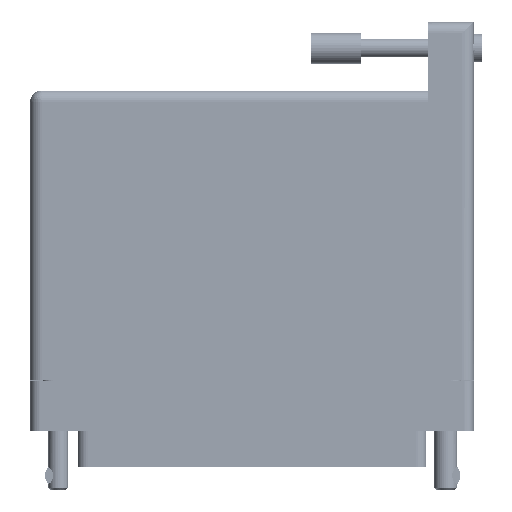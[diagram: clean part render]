
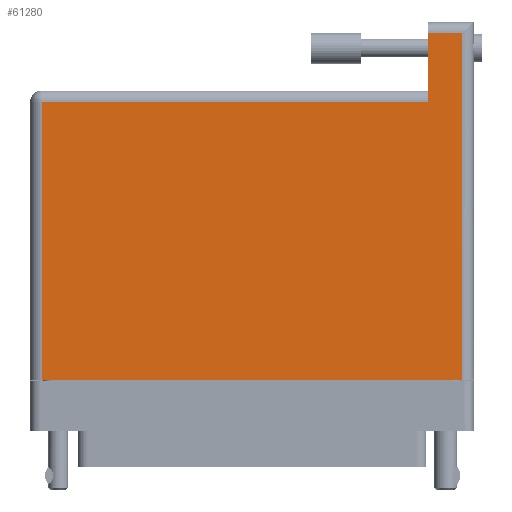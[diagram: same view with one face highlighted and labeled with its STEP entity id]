
A CAD part, front view. The second image highlights one B-rep face of the part: STEP entity #61280.
In plain terms, the highlighted face is planar.
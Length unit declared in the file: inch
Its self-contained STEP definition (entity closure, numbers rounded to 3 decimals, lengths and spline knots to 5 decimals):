
#1107 = VECTOR ( 'NONE', #55226, 39.37008 ) ;
#3086 = FACE_OUTER_BOUND ( 'NONE', #18941, .T. ) ;
#3192 = CARTESIAN_POINT ( 'NONE',  ( -1.359, 2.025, 0.617 ) ) ;
#4918 = DIRECTION ( 'NONE',  ( 1., 0., 0. ) ) ;
#5148 = LINE ( 'NONE', #23164, #1107 ) ;
#5359 = EDGE_CURVE ( 'NONE', #36447, #42896, #19551, .T. ) ;
#5602 = CARTESIAN_POINT ( 'NONE',  ( 1.289, 2.095, 0.617 ) ) ;
#7610 = VERTEX_POINT ( 'NONE', #39998 ) ;
#8153 = VECTOR ( 'NONE', #71658, 39.37008 ) ;
#9639 = LINE ( 'NONE', #28897, #49047 ) ;
#10037 = ORIENTED_EDGE ( 'NONE', *, *, #51662, .T. ) ;
#11265 = CARTESIAN_POINT ( 'NONE',  ( 1.289, -0.1, 0.617 ) ) ;
#13018 = CARTESIAN_POINT ( 'NONE',  ( 1.289, 2.025, 0.617 ) ) ;
#13478 = CARTESIAN_POINT ( 'NONE',  ( 1.079, 1.605, 0.617 ) ) ;
#14288 = VERTEX_POINT ( 'NONE', #25095 ) ;
#18941 = EDGE_LOOP ( 'NONE', ( #81560, #20377, #53331, #40989, #45799, #10037 ) ) ;
#19291 = EDGE_CURVE ( 'NONE', #76613, #59127, #5148, .T. ) ;
#19497 = CARTESIAN_POINT ( 'NONE',  ( 1.079, 2.095, 0.617 ) ) ;
#19551 = LINE ( 'NONE', #5602, #54060 ) ;
#20377 = ORIENTED_EDGE ( 'NONE', *, *, #80144, .T. ) ;
#21695 = PLANE ( 'NONE',  #30352 ) ;
#22067 = CARTESIAN_POINT ( 'NONE',  ( -1.289, -0.1, 0.617 ) ) ;
#23164 = CARTESIAN_POINT ( 'NONE',  ( -1.359, 1.605, 0.617 ) ) ;
#25095 = CARTESIAN_POINT ( 'NONE',  ( -1.289, -0.1, 0.617 ) ) ;
#25992 = EDGE_CURVE ( 'NONE', #42896, #7610, #26739, .T. ) ;
#26739 = LINE ( 'NONE', #3192, #75438 ) ;
#28897 = CARTESIAN_POINT ( 'NONE',  ( -1.359, -0.1, 0.617 ) ) ;
#30352 = AXIS2_PLACEMENT_3D ( 'NONE', #80577, #67084, #67638 ) ;
#36447 = VERTEX_POINT ( 'NONE', #11265 ) ;
#39998 = CARTESIAN_POINT ( 'NONE',  ( 1.079, 2.025, 0.617 ) ) ;
#40989 = ORIENTED_EDGE ( 'NONE', *, *, #5359, .T. ) ;
#42896 = VERTEX_POINT ( 'NONE', #13018 ) ;
#45799 = ORIENTED_EDGE ( 'NONE', *, *, #25992, .T. ) ;
#46057 = LINE ( 'NONE', #22067, #49146 ) ;
#47373 = CARTESIAN_POINT ( 'NONE',  ( -1.289, 1.605, 0.617 ) ) ;
#47644 = LINE ( 'NONE', #19497, #8153 ) ;
#49047 = VECTOR ( 'NONE', #4918, 39.37008 ) ;
#49146 = VECTOR ( 'NONE', #66594, 39.37008 ) ;
#51662 = EDGE_CURVE ( 'NONE', #7610, #76613, #47644, .T. ) ;
#53331 = ORIENTED_EDGE ( 'NONE', *, *, #79670, .T. ) ;
#54060 = VECTOR ( 'NONE', #64473, 39.37008 ) ;
#55226 = DIRECTION ( 'NONE',  ( -1., 0., 0. ) ) ;
#59127 = VERTEX_POINT ( 'NONE', #47373 ) ;
#61280 = ADVANCED_FACE ( 'NONE', ( #3086 ), #21695, .F. ) ;
#61464 = DIRECTION ( 'NONE',  ( -1., 0., 0. ) ) ;
#64473 = DIRECTION ( 'NONE',  ( 0., 1., 0. ) ) ;
#66594 = DIRECTION ( 'NONE',  ( 0., -1., 0. ) ) ;
#67084 = DIRECTION ( 'NONE',  ( 0., 0., -1. ) ) ;
#67638 = DIRECTION ( 'NONE',  ( -1., 0., 0. ) ) ;
#71658 = DIRECTION ( 'NONE',  ( 0., -1., 0. ) ) ;
#75438 = VECTOR ( 'NONE', #61464, 39.37008 ) ;
#76613 = VERTEX_POINT ( 'NONE', #13478 ) ;
#79670 = EDGE_CURVE ( 'NONE', #14288, #36447, #9639, .T. ) ;
#80144 = EDGE_CURVE ( 'NONE', #59127, #14288, #46057, .T. ) ;
#80577 = CARTESIAN_POINT ( 'NONE',  ( -1.359, 1.675, 0.617 ) ) ;
#81560 = ORIENTED_EDGE ( 'NONE', *, *, #19291, .T. ) ;
